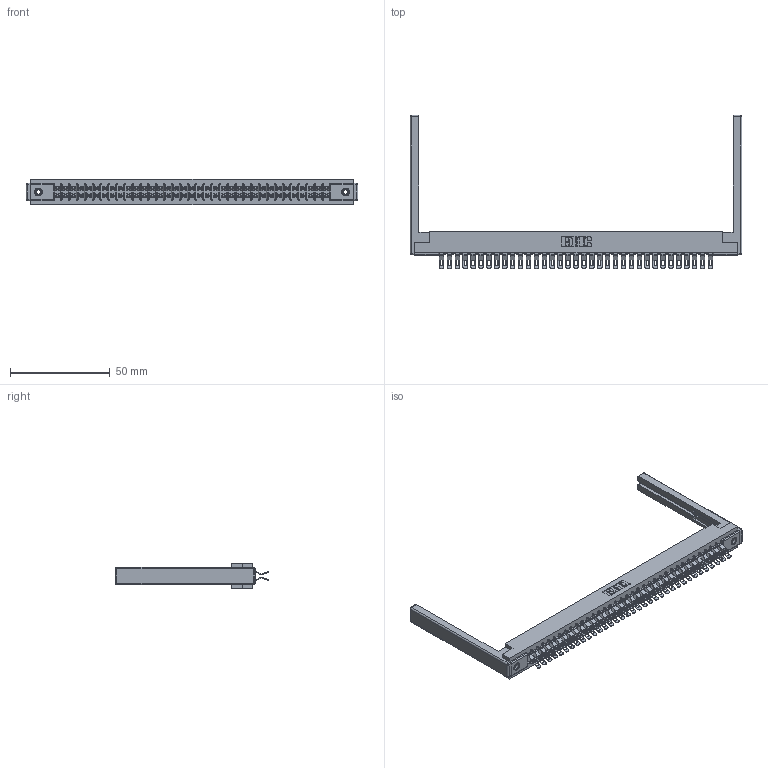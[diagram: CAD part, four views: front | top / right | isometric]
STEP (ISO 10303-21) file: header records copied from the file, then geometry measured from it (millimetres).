
FILE_DESCRIPTION (( 'STEP AP203' ), '1' );
FILE_NAME ('307-070-455-268.STEP', '2020-10-01T00:31:11', ( '' ), ( '' ), 'SwSTEP 2.0', 'SolidWorks 2020', '' );
FILE_SCHEMA (( 'CONFIG_CONTROL_DESIGN' ));
Length unit declared in the file: inch
Products named in the file (5): 307-220-068; 307-070-455-268; 345-250-001_345-250-001-102; 307 Part_.156 Dia Mounting Holes; 307-290-001_555
Assembly tree (75 placements, depth 2):
  307-070-455-268
    307 Part_.156 Dia Mounting Holes
    307-290-001_555  x70
    307-220-068  x2
    345-250-001_345-250-001-102  x2
Bounding box: 166.12 x 76.71 x 12.7 mm (x, y, z)
Volume: 22204 mm3; surface area: 26806.2 mm2
Topology: 75 solids, 75 shells, 4578 faces, 13383 edges, 8710 vertices
Faces by surface type: plane 2538, cylinder 1944, sphere 80, cone 12, torus 4
Entity records: 35284 total; most frequent: CARTESIAN_POINT 5756, ORIENTED_EDGE 5698, DIRECTION 5663, EDGE_CURVE 2849, VECTOR 2169, LINE 2169, VERTEX_POINT 1840, AXIS2_PLACEMENT_3D 1747
